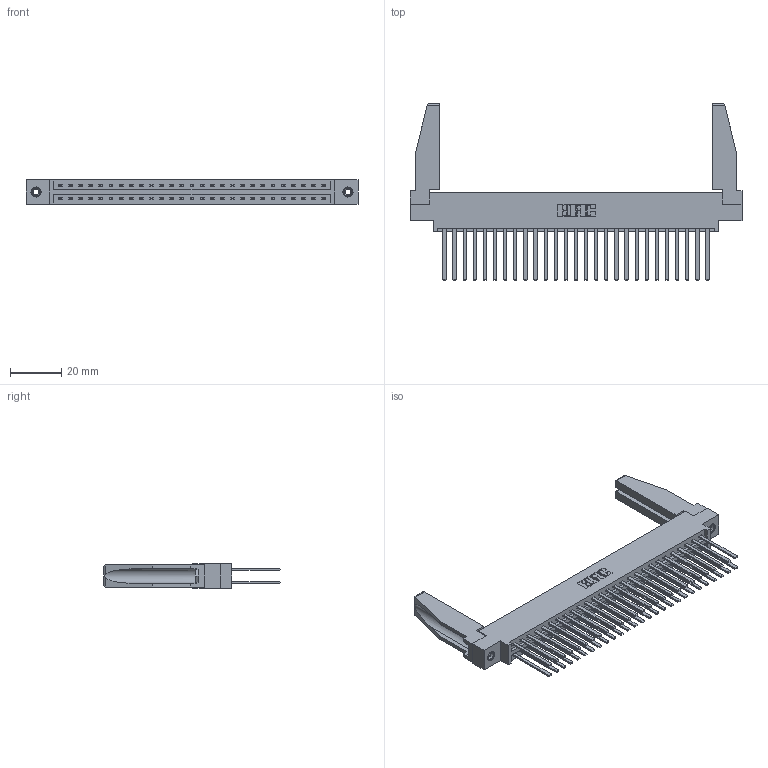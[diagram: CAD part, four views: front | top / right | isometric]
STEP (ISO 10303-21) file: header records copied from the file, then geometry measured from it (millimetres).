
FILE_DESCRIPTION (( 'STEP AP203' ), '1' );
FILE_NAME ('387-054-544-878.STEP', '2019-10-19T05:23:21', ( '' ), ( '' ), 'SwSTEP 2.0', 'SolidWorks 2016', '' );
FILE_SCHEMA (( 'CONFIG_CONTROL_DESIGN' ));
Length unit declared in the file: inch
Products named in the file (5): 307-220-078; 345-292-001_345-293-144; 345-250-001_345-250-001-102; 387-054-544-878; 337 Part_0.170 Offset - 0.156 Dia-TI
Assembly tree (59 placements, depth 2):
  387-054-544-878
    337 Part_0.170 Offset - 0.156 Dia-TI
    345-292-001_345-293-144  x54
    345-250-001_345-250-001-102  x2
    307-220-078  x2
Bounding box: 130 x 69.09 x 9.4 mm (x, y, z)
Volume: 18133.3 mm3; surface area: 22250.7 mm2
Topology: 59 solids, 59 shells, 2840 faces, 8375 edges, 5502 vertices
Faces by surface type: plane 1994, cylinder 830, cone 12, torus 4
Entity records: 25262 total; most frequent: CARTESIAN_POINT 4268, ORIENTED_EDGE 4160, DIRECTION 3660, EDGE_CURVE 2080, VECTOR 1918, LINE 1918, VERTEX_POINT 1380, AXIS2_PLACEMENT_3D 871
